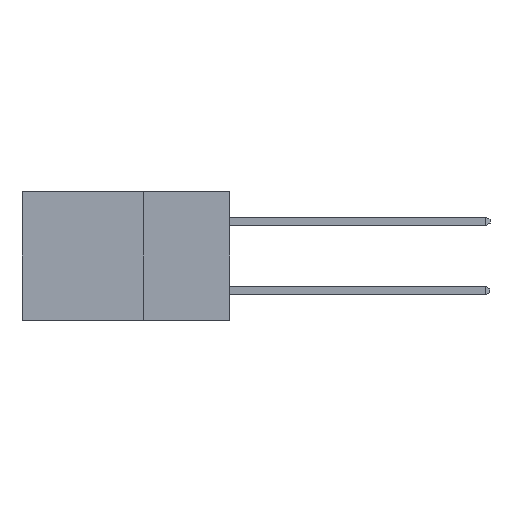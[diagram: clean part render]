
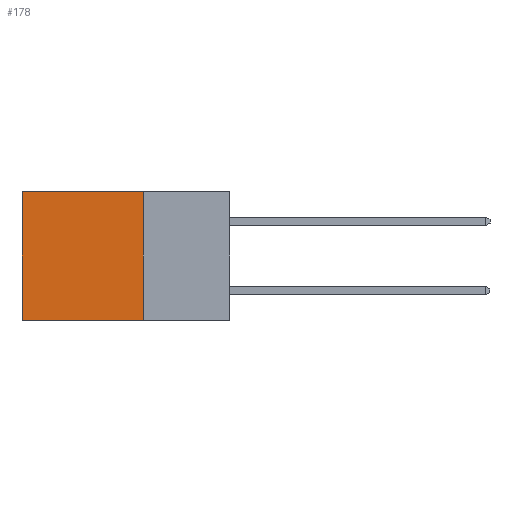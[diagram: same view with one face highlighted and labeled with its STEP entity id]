
A CAD part, left-side view. The second image highlights one B-rep face of the part: STEP entity #178.
In plain terms, the highlighted planar face has unit normal (-1, 0, 0).
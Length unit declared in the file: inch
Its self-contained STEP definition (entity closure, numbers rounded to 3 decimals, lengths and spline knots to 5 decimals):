
#118 = LINE ( 'NONE', #18364, #695 ) ;
#178 = ADVANCED_FACE ( 'NONE', ( #21537 ), #21316, .F. ) ;
#695 = VECTOR ( 'NONE', #7178, 39.37008 ) ;
#729 = CARTESIAN_POINT ( 'NONE',  ( 0.298, 0.6, 0. ) ) ;
#1083 = EDGE_CURVE ( 'NONE', #10086, #7576, #12693, .T. ) ;
#2484 = EDGE_CURVE ( 'NONE', #20204, #3739, #24025, .T. ) ;
#2787 = CARTESIAN_POINT ( 'NONE',  ( 0.298, 0.25, 0. ) ) ;
#3071 = LINE ( 'NONE', #12351, #22275 ) ;
#3739 = VERTEX_POINT ( 'NONE', #14989 ) ;
#3896 = ORIENTED_EDGE ( 'NONE', *, *, #1083, .T. ) ;
#4603 = ORIENTED_EDGE ( 'NONE', *, *, #19628, .F. ) ;
#6215 = CARTESIAN_POINT ( 'NONE',  ( 0.298, 0.6, -0.37 ) ) ;
#6625 = ORIENTED_EDGE ( 'NONE', *, *, #8423, .T. ) ;
#7178 = DIRECTION ( 'NONE',  ( 0., 1., 0. ) ) ;
#7576 = VERTEX_POINT ( 'NONE', #6215 ) ;
#8423 = EDGE_CURVE ( 'NONE', #20204, #10086, #118, .T. ) ;
#10086 = VERTEX_POINT ( 'NONE', #729 ) ;
#12351 = CARTESIAN_POINT ( 'NONE',  ( 0.298, 0.25, -0.37 ) ) ;
#12693 = LINE ( 'NONE', #20300, #20887 ) ;
#13420 = EDGE_LOOP ( 'NONE', ( #3896, #4603, #14877, #6625 ) ) ;
#14011 = DIRECTION ( 'NONE',  ( 0., 0., -1. ) ) ;
#14081 = VECTOR ( 'NONE', #14011, 39.37008 ) ;
#14877 = ORIENTED_EDGE ( 'NONE', *, *, #2484, .F. ) ;
#14989 = CARTESIAN_POINT ( 'NONE',  ( 0.298, 0.25, -0.37 ) ) ;
#16434 = CARTESIAN_POINT ( 'NONE',  ( 0.298, 0.25, 0. ) ) ;
#16512 = AXIS2_PLACEMENT_3D ( 'NONE', #16434, #21246, #21013 ) ;
#16926 = CARTESIAN_POINT ( 'NONE',  ( 0.298, 0.25, 0. ) ) ;
#18027 = DIRECTION ( 'NONE',  ( 0., 1., 0. ) ) ;
#18364 = CARTESIAN_POINT ( 'NONE',  ( 0.298, 0.25, 0. ) ) ;
#19628 = EDGE_CURVE ( 'NONE', #3739, #7576, #3071, .T. ) ;
#20204 = VERTEX_POINT ( 'NONE', #2787 ) ;
#20300 = CARTESIAN_POINT ( 'NONE',  ( 0.298, 0.6, 0. ) ) ;
#20662 = DIRECTION ( 'NONE',  ( 0., 0., -1. ) ) ;
#20887 = VECTOR ( 'NONE', #20662, 39.37008 ) ;
#21013 = DIRECTION ( 'NONE',  ( 0., 0., -1. ) ) ;
#21246 = DIRECTION ( 'NONE',  ( 1., 0., 0. ) ) ;
#21316 = PLANE ( 'NONE',  #16512 ) ;
#21537 = FACE_OUTER_BOUND ( 'NONE', #13420, .T. ) ;
#22275 = VECTOR ( 'NONE', #18027, 39.37008 ) ;
#24025 = LINE ( 'NONE', #16926, #14081 ) ;
